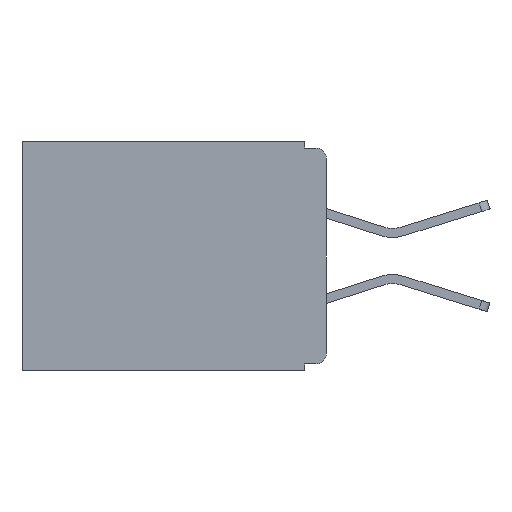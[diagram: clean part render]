
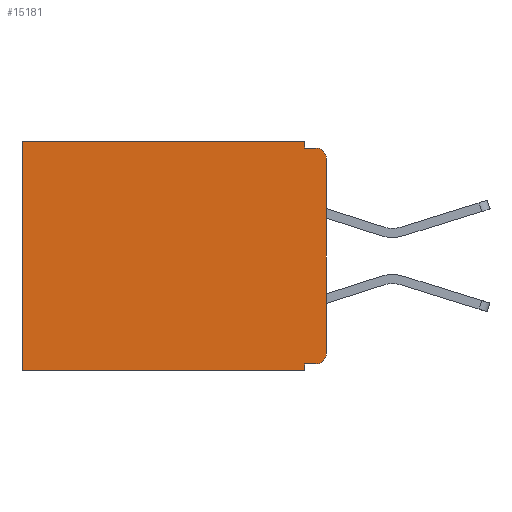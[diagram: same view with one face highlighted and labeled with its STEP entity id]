
A CAD part, left-side view. The second image highlights one B-rep face of the part: STEP entity #15181.
In plain terms, the highlighted planar face has unit normal (-1, 0, 0).
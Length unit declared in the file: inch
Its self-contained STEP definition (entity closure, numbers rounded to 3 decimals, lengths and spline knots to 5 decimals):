
#260 = CARTESIAN_POINT ( 'NONE',  ( 0.3, 0.015, -0.025 ) ) ;
#663 = DIRECTION ( 'NONE',  ( -1., 0., 0. ) ) ;
#763 = DIRECTION ( 'NONE',  ( 0., 0., -1. ) ) ;
#890 = CARTESIAN_POINT ( 'NONE',  ( 0.3, 0.031, 0. ) ) ;
#1141 = CARTESIAN_POINT ( 'NONE',  ( 0.3, 0.015, -0.32 ) ) ;
#1814 = EDGE_CURVE ( 'NONE', #2049, #17882, #9917, .T. ) ;
#2005 = VECTOR ( 'NONE', #26439, 39.37008 ) ;
#2049 = VERTEX_POINT ( 'NONE', #12508 ) ;
#2194 = EDGE_CURVE ( 'NONE', #24038, #12118, #18142, .T. ) ;
#2259 = DIRECTION ( 'NONE',  ( 0., 0., -1. ) ) ;
#3145 = VERTEX_POINT ( 'NONE', #5208 ) ;
#3784 = VECTOR ( 'NONE', #19756, 39.37008 ) ;
#4176 = DIRECTION ( 'NONE',  ( 0., -1., 0. ) ) ;
#4789 = LINE ( 'NONE', #20435, #15399 ) ;
#5002 = VERTEX_POINT ( 'NONE', #10060 ) ;
#5208 = CARTESIAN_POINT ( 'NONE',  ( 0.3, 0.437, 0. ) ) ;
#5672 = VECTOR ( 'NONE', #17455, 39.37008 ) ;
#6254 = DIRECTION ( 'NONE',  ( 1., 0., 0. ) ) ;
#6357 = CARTESIAN_POINT ( 'NONE',  ( 0.3, 0.031, -0.32 ) ) ;
#6393 = VERTEX_POINT ( 'NONE', #6357 ) ;
#6521 = EDGE_CURVE ( 'NONE', #5002, #16605, #19258, .T. ) ;
#9095 = VECTOR ( 'NONE', #23437, 39.37008 ) ;
#9330 = EDGE_CURVE ( 'NONE', #24038, #6393, #11307, .T. ) ;
#9616 = AXIS2_PLACEMENT_3D ( 'NONE', #10433, #6254, #20930 ) ;
#9917 = LINE ( 'NONE', #12903, #20392 ) ;
#10060 = CARTESIAN_POINT ( 'NONE',  ( 0.3, 0., -0.025 ) ) ;
#10154 = CARTESIAN_POINT ( 'NONE',  ( 0.3, 0.015, -0.305 ) ) ;
#10433 = CARTESIAN_POINT ( 'NONE',  ( 0.3, 0., -0.33 ) ) ;
#10453 = LINE ( 'NONE', #13041, #9095 ) ;
#10740 = AXIS2_PLACEMENT_3D ( 'NONE', #260, #663, #24103 ) ;
#11307 = LINE ( 'NONE', #25479, #5672 ) ;
#12118 = VERTEX_POINT ( 'NONE', #24926 ) ;
#12452 = VECTOR ( 'NONE', #763, 39.37008 ) ;
#12508 = CARTESIAN_POINT ( 'NONE',  ( 0.3, 0.031, -0.33 ) ) ;
#12534 = PLANE ( 'NONE',  #9616 ) ;
#12597 = CARTESIAN_POINT ( 'NONE',  ( 0.3, 0., -0.01 ) ) ;
#12903 = CARTESIAN_POINT ( 'NONE',  ( 0.3, 0., -0.33 ) ) ;
#13041 = CARTESIAN_POINT ( 'NONE',  ( 0.3, 0.031, -0.33 ) ) ;
#13224 = FACE_OUTER_BOUND ( 'NONE', #16274, .T. ) ;
#14014 = AXIS2_PLACEMENT_3D ( 'NONE', #10154, #25505, #2259 ) ;
#15181 = ADVANCED_FACE ( 'NONE', ( #13224 ), #12534, .F. ) ;
#15399 = VECTOR ( 'NONE', #22474, 39.37008 ) ;
#16274 = EDGE_LOOP ( 'NONE', ( #21551, #22156, #22516, #22537, #23371, #23401, #24052, #24315, #24368, #24642 ) ) ;
#16605 = VERTEX_POINT ( 'NONE', #19179 ) ;
#17455 = DIRECTION ( 'NONE',  ( 0., 1., 0. ) ) ;
#17470 = EDGE_CURVE ( 'NONE', #3145, #17882, #24068, .T. ) ;
#17696 = CARTESIAN_POINT ( 'NONE',  ( 0.3, 0., 0. ) ) ;
#17838 = EDGE_CURVE ( 'NONE', #19768, #16605, #24043, .T. ) ;
#17882 = VERTEX_POINT ( 'NONE', #25026 ) ;
#18002 = EDGE_CURVE ( 'NONE', #6393, #2049, #10453, .T. ) ;
#18042 = CARTESIAN_POINT ( 'NONE',  ( 0.3, 0.031, -0.01 ) ) ;
#18142 = CIRCLE ( 'NONE', #14014, 0.015 ) ;
#18682 = VECTOR ( 'NONE', #4176, 39.37008 ) ;
#18916 = LINE ( 'NONE', #24496, #2005 ) ;
#19179 = CARTESIAN_POINT ( 'NONE',  ( 0.3, 0.015, -0.01 ) ) ;
#19258 = CIRCLE ( 'NONE', #10740, 0.015 ) ;
#19375 = EDGE_CURVE ( 'NONE', #20355, #19768, #18916, .T. ) ;
#19756 = DIRECTION ( 'NONE',  ( 0., 1., 0. ) ) ;
#19768 = VERTEX_POINT ( 'NONE', #18042 ) ;
#20355 = VERTEX_POINT ( 'NONE', #890 ) ;
#20392 = VECTOR ( 'NONE', #24054, 39.37008 ) ;
#20435 = CARTESIAN_POINT ( 'NONE',  ( 0.3, 0., -0.33 ) ) ;
#20582 = LINE ( 'NONE', #17696, #3784 ) ;
#20930 = DIRECTION ( 'NONE',  ( 0., 0., -1. ) ) ;
#21551 = ORIENTED_EDGE ( 'NONE', *, *, #24620, .F. ) ;
#22156 = ORIENTED_EDGE ( 'NONE', *, *, #6521, .T. ) ;
#22474 = DIRECTION ( 'NONE',  ( 0., 0., -1. ) ) ;
#22516 = ORIENTED_EDGE ( 'NONE', *, *, #17838, .F. ) ;
#22537 = ORIENTED_EDGE ( 'NONE', *, *, #19375, .F. ) ;
#23371 = ORIENTED_EDGE ( 'NONE', *, *, #24891, .T. ) ;
#23401 = ORIENTED_EDGE ( 'NONE', *, *, #17470, .T. ) ;
#23437 = DIRECTION ( 'NONE',  ( 0., 0., -1. ) ) ;
#23804 = CARTESIAN_POINT ( 'NONE',  ( 0.3, 0.437, -0.33 ) ) ;
#24038 = VERTEX_POINT ( 'NONE', #1141 ) ;
#24043 = LINE ( 'NONE', #12597, #18682 ) ;
#24052 = ORIENTED_EDGE ( 'NONE', *, *, #1814, .F. ) ;
#24054 = DIRECTION ( 'NONE',  ( 0., 1., 0. ) ) ;
#24068 = LINE ( 'NONE', #23804, #12452 ) ;
#24103 = DIRECTION ( 'NONE',  ( 0., 0., -1. ) ) ;
#24315 = ORIENTED_EDGE ( 'NONE', *, *, #18002, .F. ) ;
#24368 = ORIENTED_EDGE ( 'NONE', *, *, #9330, .F. ) ;
#24496 = CARTESIAN_POINT ( 'NONE',  ( 0.3, 0.031, 0. ) ) ;
#24620 = EDGE_CURVE ( 'NONE', #5002, #12118, #4789, .T. ) ;
#24642 = ORIENTED_EDGE ( 'NONE', *, *, #2194, .T. ) ;
#24891 = EDGE_CURVE ( 'NONE', #20355, #3145, #20582, .T. ) ;
#24926 = CARTESIAN_POINT ( 'NONE',  ( 0.3, 0., -0.305 ) ) ;
#25026 = CARTESIAN_POINT ( 'NONE',  ( 0.3, 0.437, -0.33 ) ) ;
#25479 = CARTESIAN_POINT ( 'NONE',  ( 0.3, 0., -0.32 ) ) ;
#25505 = DIRECTION ( 'NONE',  ( -1., 0., 0. ) ) ;
#26439 = DIRECTION ( 'NONE',  ( 0., 0., -1. ) ) ;
